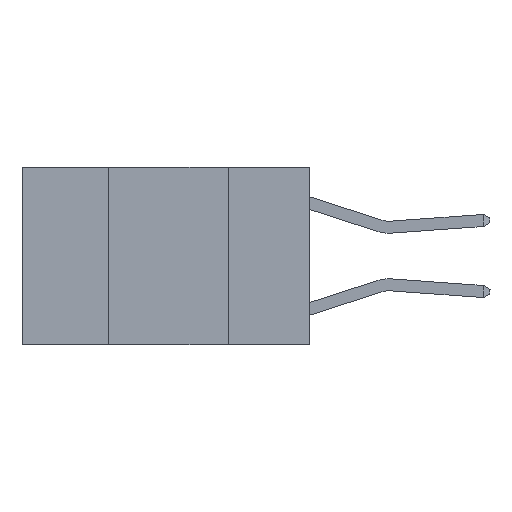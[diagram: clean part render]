
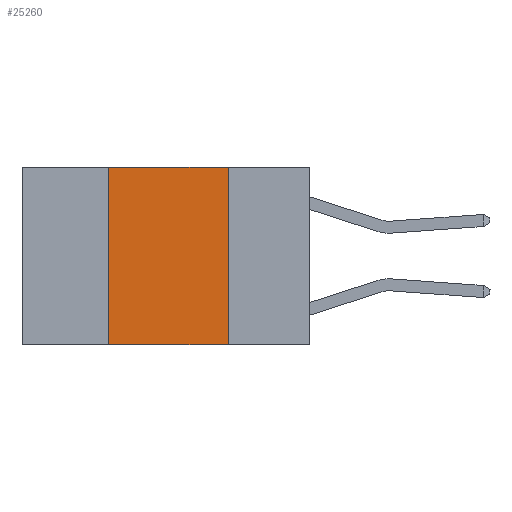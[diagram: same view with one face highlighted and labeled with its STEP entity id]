
A CAD part, left-side view. The second image highlights one B-rep face of the part: STEP entity #25260.
In plain terms, the highlighted planar face has unit normal (-1, 0, 0).
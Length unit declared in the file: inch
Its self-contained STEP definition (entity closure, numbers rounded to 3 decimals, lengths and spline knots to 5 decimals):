
#776 = EDGE_CURVE ( 'NONE', #27840, #26063, #12404, .T. ) ;
#1530 = LINE ( 'NONE', #20714, #8194 ) ;
#1606 = DIRECTION ( 'NONE',  ( 0., 0., -1. ) ) ;
#1654 = CARTESIAN_POINT ( 'NONE',  ( 0., 0.6, -0.37 ) ) ;
#2486 = EDGE_CURVE ( 'NONE', #12095, #29810, #11560, .T. ) ;
#2681 = CARTESIAN_POINT ( 'NONE',  ( 0., 0.6, 0. ) ) ;
#5590 = ORIENTED_EDGE ( 'NONE', *, *, #22379, .T. ) ;
#5891 = DIRECTION ( 'NONE',  ( 0., -1., 0. ) ) ;
#6488 = VECTOR ( 'NONE', #1606, 39.37008 ) ;
#7351 = VECTOR ( 'NONE', #29255, 39.37008 ) ;
#7712 = DIRECTION ( 'NONE',  ( 0., 0., -1. ) ) ;
#8194 = VECTOR ( 'NONE', #5891, 39.37008 ) ;
#8322 = CARTESIAN_POINT ( 'NONE',  ( 0., 0.42, 0. ) ) ;
#9917 = ORIENTED_EDGE ( 'NONE', *, *, #19406, .F. ) ;
#11560 = LINE ( 'NONE', #16531, #6488 ) ;
#12095 = VERTEX_POINT ( 'NONE', #26432 ) ;
#12404 = LINE ( 'NONE', #20856, #7351 ) ;
#12802 = EDGE_LOOP ( 'NONE', ( #22208, #9917, #24500, #5590 ) ) ;
#13439 = LINE ( 'NONE', #1654, #18443 ) ;
#16531 = CARTESIAN_POINT ( 'NONE',  ( 0., 0.17, 0. ) ) ;
#18443 = VECTOR ( 'NONE', #21481, 39.37008 ) ;
#18741 = CARTESIAN_POINT ( 'NONE',  ( 0., 0.42, -0.37 ) ) ;
#19406 = EDGE_CURVE ( 'NONE', #26063, #12095, #1530, .T. ) ;
#20019 = PLANE ( 'NONE',  #20256 ) ;
#20256 = AXIS2_PLACEMENT_3D ( 'NONE', #2681, #22457, #7712 ) ;
#20714 = CARTESIAN_POINT ( 'NONE',  ( 0., 0.6, 0. ) ) ;
#20856 = CARTESIAN_POINT ( 'NONE',  ( 0., 0.42, 0. ) ) ;
#21019 = CARTESIAN_POINT ( 'NONE',  ( 0., 0.17, -0.37 ) ) ;
#21481 = DIRECTION ( 'NONE',  ( 0., -1., 0. ) ) ;
#22208 = ORIENTED_EDGE ( 'NONE', *, *, #2486, .F. ) ;
#22379 = EDGE_CURVE ( 'NONE', #27840, #29810, #13439, .T. ) ;
#22457 = DIRECTION ( 'NONE',  ( 1., 0., 0. ) ) ;
#24500 = ORIENTED_EDGE ( 'NONE', *, *, #776, .F. ) ;
#25260 = ADVANCED_FACE ( 'NONE', ( #30890 ), #20019, .F. ) ;
#26063 = VERTEX_POINT ( 'NONE', #8322 ) ;
#26432 = CARTESIAN_POINT ( 'NONE',  ( 0., 0.17, 0. ) ) ;
#27840 = VERTEX_POINT ( 'NONE', #18741 ) ;
#29255 = DIRECTION ( 'NONE',  ( 0., 0., 1. ) ) ;
#29810 = VERTEX_POINT ( 'NONE', #21019 ) ;
#30890 = FACE_OUTER_BOUND ( 'NONE', #12802, .T. ) ;
